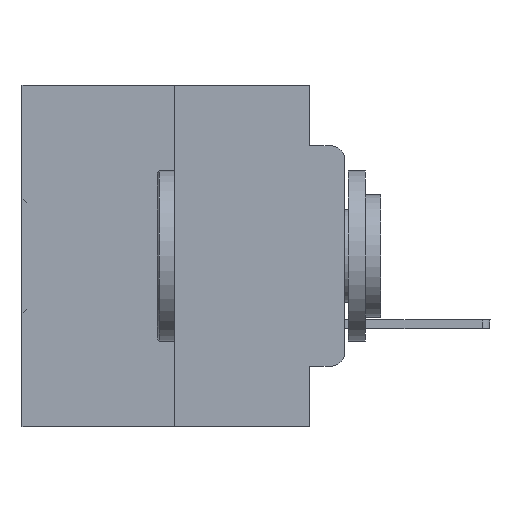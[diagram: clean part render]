
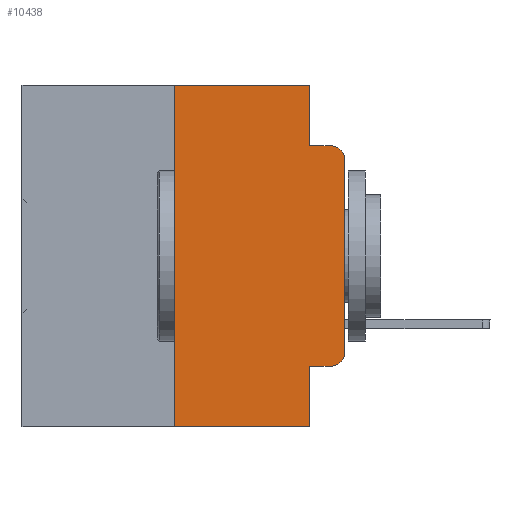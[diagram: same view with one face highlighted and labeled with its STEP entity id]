
A CAD part, left-side view. The second image highlights one B-rep face of the part: STEP entity #10438.
In plain terms, the highlighted planar face has unit normal (-1, 0, 0).
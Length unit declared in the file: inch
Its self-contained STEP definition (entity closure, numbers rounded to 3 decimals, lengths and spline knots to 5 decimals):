
#135 = AXIS2_PLACEMENT_3D ( 'NONE', #15506, #25571, #7911 ) ;
#159 = DIRECTION ( 'NONE',  ( 0., -1., 0. ) ) ;
#482 = EDGE_CURVE ( 'NONE', #23497, #4919, #12368, .T. ) ;
#669 = EDGE_CURVE ( 'NONE', #26591, #31102, #12784, .T. ) ;
#932 = CARTESIAN_POINT ( 'NONE',  ( 0., 0.25, -0.5 ) ) ;
#1067 = CARTESIAN_POINT ( 'NONE',  ( 0., 0., -0.3915 ) ) ;
#1486 = ORIENTED_EDGE ( 'NONE', *, *, #13811, .F. ) ;
#1754 = LINE ( 'NONE', #29806, #28741 ) ;
#2910 = PLANE ( 'NONE',  #8337 ) ;
#2958 = ORIENTED_EDGE ( 'NONE', *, *, #482, .F. ) ;
#3337 = DIRECTION ( 'NONE',  ( 0., -1., 0. ) ) ;
#4039 = VECTOR ( 'NONE', #3337, 39.37008 ) ;
#4486 = EDGE_LOOP ( 'NONE', ( #20354, #14483, #18921, #1486, #2958, #19821, #10628, #28171, #7019, #32285 ) ) ;
#4629 = CARTESIAN_POINT ( 'NONE',  ( 0., 0.051, -0.4115 ) ) ;
#4919 = VERTEX_POINT ( 'NONE', #25521 ) ;
#5102 = EDGE_CURVE ( 'NONE', #19019, #25242, #14919, .T. ) ;
#5392 = CARTESIAN_POINT ( 'NONE',  ( 0., 0.473, 0. ) ) ;
#5553 = FACE_OUTER_BOUND ( 'NONE', #4486, .T. ) ;
#7019 = ORIENTED_EDGE ( 'NONE', *, *, #14172, .T. ) ;
#7161 = CARTESIAN_POINT ( 'NONE',  ( 0., 0.051, 0. ) ) ;
#7361 = CARTESIAN_POINT ( 'NONE',  ( 0., 0.02, -0.0885 ) ) ;
#7911 = DIRECTION ( 'NONE',  ( 0., 0., -1. ) ) ;
#8172 = DIRECTION ( 'NONE',  ( 0., 0., 1. ) ) ;
#8337 = AXIS2_PLACEMENT_3D ( 'NONE', #5392, #24891, #12969 ) ;
#8341 = VECTOR ( 'NONE', #15077, 39.37008 ) ;
#10438 = ADVANCED_FACE ( 'NONE', ( #5553 ), #2910, .F. ) ;
#10628 = ORIENTED_EDGE ( 'NONE', *, *, #21471, .T. ) ;
#10907 = LINE ( 'NONE', #25949, #4039 ) ;
#11034 = VECTOR ( 'NONE', #159, 39.37008 ) ;
#11941 = EDGE_CURVE ( 'NONE', #18514, #29512, #31828, .T. ) ;
#12132 = CARTESIAN_POINT ( 'NONE',  ( 0., 0.02, -0.1085 ) ) ;
#12368 = LINE ( 'NONE', #24602, #11034 ) ;
#12784 = CIRCLE ( 'NONE', #135, 0.02 ) ;
#12969 = DIRECTION ( 'NONE',  ( 0., 0., -1. ) ) ;
#13696 = VERTEX_POINT ( 'NONE', #932 ) ;
#13811 = EDGE_CURVE ( 'NONE', #4919, #20401, #1754, .T. ) ;
#14024 = CARTESIAN_POINT ( 'NONE',  ( 0., 0.051, -0.0885 ) ) ;
#14172 = EDGE_CURVE ( 'NONE', #19019, #26591, #20158, .T. ) ;
#14483 = ORIENTED_EDGE ( 'NONE', *, *, #11941, .T. ) ;
#14919 = LINE ( 'NONE', #7161, #8341 ) ;
#15032 = DIRECTION ( 'NONE',  ( 0., -1., 0. ) ) ;
#15034 = EDGE_CURVE ( 'NONE', #20401, #29512, #10907, .T. ) ;
#15077 = DIRECTION ( 'NONE',  ( 0., 0., -1. ) ) ;
#15506 = CARTESIAN_POINT ( 'NONE',  ( 0., 0.02, -0.3915 ) ) ;
#15597 = LINE ( 'NONE', #18411, #23548 ) ;
#15763 = DIRECTION ( 'NONE',  ( 0., 0., 1. ) ) ;
#16542 = AXIS2_PLACEMENT_3D ( 'NONE', #12132, #22211, #21728 ) ;
#17911 = CARTESIAN_POINT ( 'NONE',  ( 0., 0., 0. ) ) ;
#18411 = CARTESIAN_POINT ( 'NONE',  ( 0., 0.25, 0. ) ) ;
#18514 = VERTEX_POINT ( 'NONE', #29660 ) ;
#18818 = EDGE_CURVE ( 'NONE', #13696, #23497, #15597, .T. ) ;
#18921 = ORIENTED_EDGE ( 'NONE', *, *, #15034, .F. ) ;
#19019 = VERTEX_POINT ( 'NONE', #20019 ) ;
#19391 = EDGE_CURVE ( 'NONE', #31102, #18514, #26005, .T. ) ;
#19821 = ORIENTED_EDGE ( 'NONE', *, *, #18818, .F. ) ;
#20019 = CARTESIAN_POINT ( 'NONE',  ( 0., 0.051, -0.4115 ) ) ;
#20158 = LINE ( 'NONE', #4629, #27705 ) ;
#20166 = LINE ( 'NONE', #25932, #22320 ) ;
#20354 = ORIENTED_EDGE ( 'NONE', *, *, #19391, .T. ) ;
#20401 = VERTEX_POINT ( 'NONE', #14024 ) ;
#21471 = EDGE_CURVE ( 'NONE', #13696, #25242, #20166, .T. ) ;
#21728 = DIRECTION ( 'NONE',  ( 0., 0., -1. ) ) ;
#22211 = DIRECTION ( 'NONE',  ( -1., 0., 0. ) ) ;
#22320 = VECTOR ( 'NONE', #27746, 39.37008 ) ;
#23262 = VECTOR ( 'NONE', #15763, 39.37008 ) ;
#23497 = VERTEX_POINT ( 'NONE', #29510 ) ;
#23548 = VECTOR ( 'NONE', #8172, 39.37008 ) ;
#24602 = CARTESIAN_POINT ( 'NONE',  ( 0., 0.473, 0. ) ) ;
#24891 = DIRECTION ( 'NONE',  ( 1., 0., 0. ) ) ;
#25242 = VERTEX_POINT ( 'NONE', #29790 ) ;
#25521 = CARTESIAN_POINT ( 'NONE',  ( 0., 0.051, 0. ) ) ;
#25571 = DIRECTION ( 'NONE',  ( -1., 0., 0. ) ) ;
#25932 = CARTESIAN_POINT ( 'NONE',  ( 0., 0.473, -0.5 ) ) ;
#25949 = CARTESIAN_POINT ( 'NONE',  ( 0., 0.051, -0.0885 ) ) ;
#26005 = LINE ( 'NONE', #17911, #23262 ) ;
#26591 = VERTEX_POINT ( 'NONE', #32441 ) ;
#27705 = VECTOR ( 'NONE', #15032, 39.37008 ) ;
#27746 = DIRECTION ( 'NONE',  ( 0., -1., 0. ) ) ;
#27949 = DIRECTION ( 'NONE',  ( 0., 0., -1. ) ) ;
#28171 = ORIENTED_EDGE ( 'NONE', *, *, #5102, .F. ) ;
#28741 = VECTOR ( 'NONE', #27949, 39.37008 ) ;
#29510 = CARTESIAN_POINT ( 'NONE',  ( 0., 0.25, 0. ) ) ;
#29512 = VERTEX_POINT ( 'NONE', #7361 ) ;
#29660 = CARTESIAN_POINT ( 'NONE',  ( 0., 0., -0.1085 ) ) ;
#29790 = CARTESIAN_POINT ( 'NONE',  ( 0., 0.051, -0.5 ) ) ;
#29806 = CARTESIAN_POINT ( 'NONE',  ( 0., 0.051, 0. ) ) ;
#31102 = VERTEX_POINT ( 'NONE', #1067 ) ;
#31828 = CIRCLE ( 'NONE', #16542, 0.02 ) ;
#32285 = ORIENTED_EDGE ( 'NONE', *, *, #669, .T. ) ;
#32441 = CARTESIAN_POINT ( 'NONE',  ( 0., 0.02, -0.4115 ) ) ;
